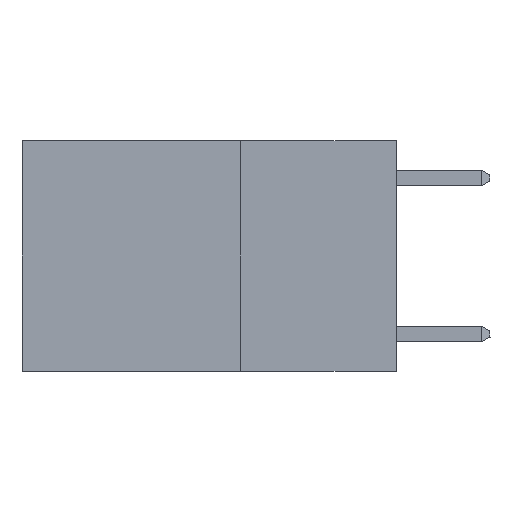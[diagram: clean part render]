
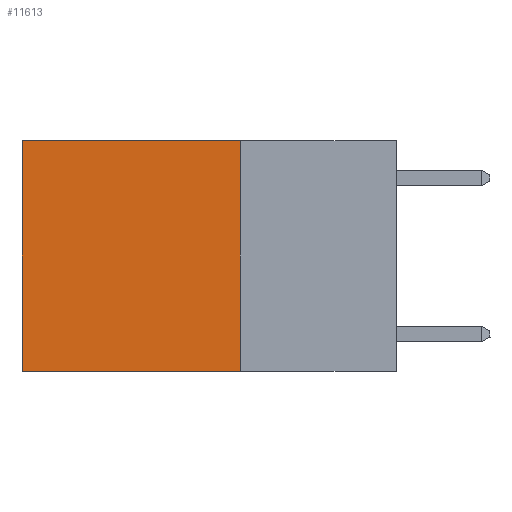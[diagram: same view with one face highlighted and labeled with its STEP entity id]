
A CAD part, left-side view. The second image highlights one B-rep face of the part: STEP entity #11613.
In plain terms, the highlighted planar face has unit normal (-1, 0, 0).
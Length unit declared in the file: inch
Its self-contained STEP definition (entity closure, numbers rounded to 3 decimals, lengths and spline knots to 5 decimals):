
#1038 = EDGE_CURVE ( 'NONE', #18529, #1774, #14405, .T. ) ;
#1774 = VERTEX_POINT ( 'NONE', #18308 ) ;
#1824 = PLANE ( 'NONE',  #16979 ) ;
#3686 = CARTESIAN_POINT ( 'NONE',  ( 0.2625, 0.25, 0. ) ) ;
#4135 = CARTESIAN_POINT ( 'NONE',  ( 0.2625, 0.25, 0. ) ) ;
#4205 = EDGE_CURVE ( 'NONE', #15667, #1774, #20755, .T. ) ;
#4734 = ORIENTED_EDGE ( 'NONE', *, *, #1038, .T. ) ;
#4798 = ORIENTED_EDGE ( 'NONE', *, *, #4205, .F. ) ;
#5181 = ORIENTED_EDGE ( 'NONE', *, *, #13769, .F. ) ;
#5268 = FACE_OUTER_BOUND ( 'NONE', #16802, .T. ) ;
#5512 = LINE ( 'NONE', #4135, #5594 ) ;
#5594 = VECTOR ( 'NONE', #16218, 39.37008 ) ;
#5999 = ORIENTED_EDGE ( 'NONE', *, *, #7427, .T. ) ;
#6470 = CARTESIAN_POINT ( 'NONE',  ( 0.2625, 0.6, 0. ) ) ;
#6959 = CARTESIAN_POINT ( 'NONE',  ( 0.2625, 0.25, -0.37 ) ) ;
#7427 = EDGE_CURVE ( 'NONE', #18838, #18529, #5512, .T. ) ;
#7512 = DIRECTION ( 'NONE',  ( 0., 0., -1. ) ) ;
#7688 = CARTESIAN_POINT ( 'NONE',  ( 0.2625, 0.6, 0. ) ) ;
#9112 = DIRECTION ( 'NONE',  ( 0., 0., -1. ) ) ;
#11608 = DIRECTION ( 'NONE',  ( 0., 1., 0. ) ) ;
#11613 = ADVANCED_FACE ( 'NONE', ( #5268 ), #1824, .F. ) ;
#11958 = LINE ( 'NONE', #20384, #12024 ) ;
#12024 = VECTOR ( 'NONE', #12435, 39.37008 ) ;
#12420 = CARTESIAN_POINT ( 'NONE',  ( 0.2625, 0.25, -0.37 ) ) ;
#12435 = DIRECTION ( 'NONE',  ( 0., 0., -1. ) ) ;
#13769 = EDGE_CURVE ( 'NONE', #18838, #15667, #11958, .T. ) ;
#14369 = VECTOR ( 'NONE', #7512, 39.37008 ) ;
#14405 = LINE ( 'NONE', #7688, #14369 ) ;
#15667 = VERTEX_POINT ( 'NONE', #6959 ) ;
#16218 = DIRECTION ( 'NONE',  ( 0., 1., 0. ) ) ;
#16802 = EDGE_LOOP ( 'NONE', ( #4734, #4798, #5181, #5999 ) ) ;
#16979 = AXIS2_PLACEMENT_3D ( 'NONE', #3686, #18903, #9112 ) ;
#18308 = CARTESIAN_POINT ( 'NONE',  ( 0.2625, 0.6, -0.37 ) ) ;
#18529 = VERTEX_POINT ( 'NONE', #6470 ) ;
#18838 = VERTEX_POINT ( 'NONE', #19082 ) ;
#18903 = DIRECTION ( 'NONE',  ( 1., 0., 0. ) ) ;
#19082 = CARTESIAN_POINT ( 'NONE',  ( 0.2625, 0.25, 0. ) ) ;
#20304 = VECTOR ( 'NONE', #11608, 39.37008 ) ;
#20384 = CARTESIAN_POINT ( 'NONE',  ( 0.2625, 0.25, 0. ) ) ;
#20755 = LINE ( 'NONE', #12420, #20304 ) ;
